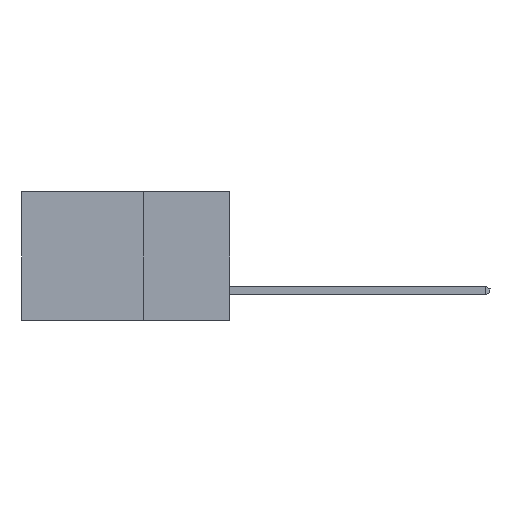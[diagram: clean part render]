
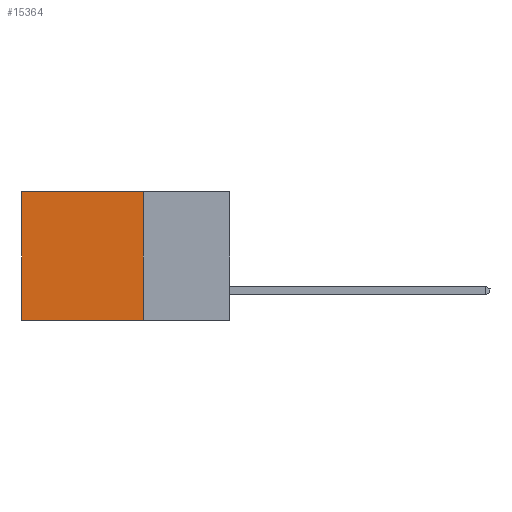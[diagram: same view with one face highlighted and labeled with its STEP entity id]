
A CAD part, left-side view. The second image highlights one B-rep face of the part: STEP entity #15364.
In plain terms, the highlighted planar face has unit normal (-1, 0, 0).
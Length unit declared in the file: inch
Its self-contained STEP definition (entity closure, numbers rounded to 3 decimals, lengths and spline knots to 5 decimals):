
#740 = FACE_OUTER_BOUND ( 'NONE', #4784, .T. ) ;
#2248 = DIRECTION ( 'NONE',  ( 0., 1., 0. ) ) ;
#2537 = DIRECTION ( 'NONE',  ( 0., 1., 0. ) ) ;
#2609 = DIRECTION ( 'NONE',  ( 0., 0., -1. ) ) ;
#2690 = VERTEX_POINT ( 'NONE', #6967 ) ;
#3100 = CARTESIAN_POINT ( 'NONE',  ( 0.2615, 0.25, 0. ) ) ;
#4479 = CARTESIAN_POINT ( 'NONE',  ( 0.2615, 0.6, 0. ) ) ;
#4784 = EDGE_LOOP ( 'NONE', ( #6867, #18204, #12715, #16041 ) ) ;
#5005 = CARTESIAN_POINT ( 'NONE',  ( 0.2615, 0.25, -0.37 ) ) ;
#5227 = LINE ( 'NONE', #19205, #24473 ) ;
#5632 = VERTEX_POINT ( 'NONE', #10050 ) ;
#6328 = EDGE_CURVE ( 'NONE', #19912, #5632, #15980, .T. ) ;
#6569 = CARTESIAN_POINT ( 'NONE',  ( 0.2615, 0.6, -0.37 ) ) ;
#6639 = LINE ( 'NONE', #17748, #11717 ) ;
#6867 = ORIENTED_EDGE ( 'NONE', *, *, #8397, .T. ) ;
#6967 = CARTESIAN_POINT ( 'NONE',  ( 0.2615, 0.6, -0.37 ) ) ;
#6990 = VECTOR ( 'NONE', #17797, 39.37008 ) ;
#8397 = EDGE_CURVE ( 'NONE', #17061, #2690, #12085, .T. ) ;
#8987 = DIRECTION ( 'NONE',  ( 0., 0., -1. ) ) ;
#10050 = CARTESIAN_POINT ( 'NONE',  ( 0.2615, 0.25, -0.37 ) ) ;
#10167 = EDGE_CURVE ( 'NONE', #5632, #2690, #6639, .T. ) ;
#11717 = VECTOR ( 'NONE', #2537, 39.37008 ) ;
#12085 = LINE ( 'NONE', #6569, #6990 ) ;
#12715 = ORIENTED_EDGE ( 'NONE', *, *, #6328, .F. ) ;
#14455 = AXIS2_PLACEMENT_3D ( 'NONE', #5005, #20143, #8987 ) ;
#15364 = ADVANCED_FACE ( 'NONE', ( #740 ), #18303, .F. ) ;
#15980 = LINE ( 'NONE', #23855, #20260 ) ;
#16041 = ORIENTED_EDGE ( 'NONE', *, *, #18293, .T. ) ;
#17061 = VERTEX_POINT ( 'NONE', #4479 ) ;
#17748 = CARTESIAN_POINT ( 'NONE',  ( 0.2615, 0.25, -0.37 ) ) ;
#17797 = DIRECTION ( 'NONE',  ( 0., 0., -1. ) ) ;
#18204 = ORIENTED_EDGE ( 'NONE', *, *, #10167, .F. ) ;
#18293 = EDGE_CURVE ( 'NONE', #19912, #17061, #5227, .T. ) ;
#18303 = PLANE ( 'NONE',  #14455 ) ;
#19205 = CARTESIAN_POINT ( 'NONE',  ( 0.2615, 0.25, 0. ) ) ;
#19912 = VERTEX_POINT ( 'NONE', #3100 ) ;
#20143 = DIRECTION ( 'NONE',  ( 1., 0., 0. ) ) ;
#20260 = VECTOR ( 'NONE', #2609, 39.37008 ) ;
#23855 = CARTESIAN_POINT ( 'NONE',  ( 0.2615, 0.25, -0.37 ) ) ;
#24473 = VECTOR ( 'NONE', #2248, 39.37008 ) ;
